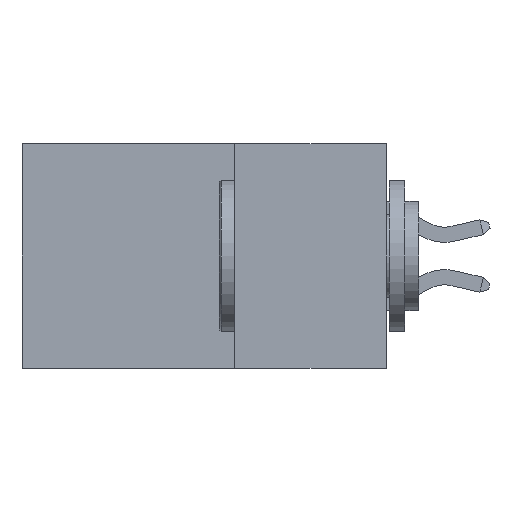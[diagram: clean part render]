
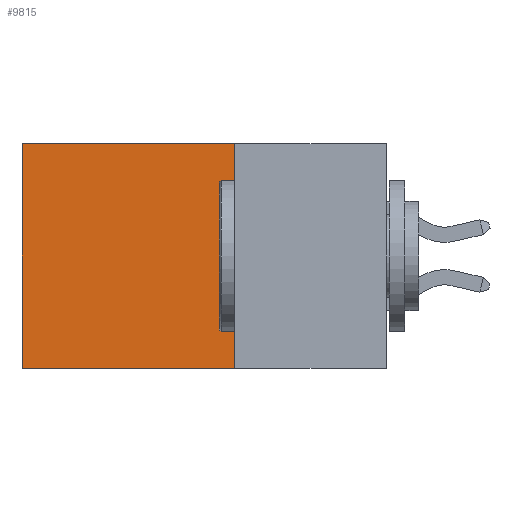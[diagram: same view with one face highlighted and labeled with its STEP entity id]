
A CAD part, left-side view. The second image highlights one B-rep face of the part: STEP entity #9815.
In plain terms, the highlighted planar face has unit normal (-1, 0, 0).
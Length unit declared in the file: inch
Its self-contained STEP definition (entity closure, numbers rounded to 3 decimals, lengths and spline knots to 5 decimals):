
#515 = EDGE_LOOP ( 'NONE', ( #5814, #2212, #3972, #2820 ) ) ;
#519 = DIRECTION ( 'NONE',  ( 0., 0., -1. ) ) ;
#528 = DIRECTION ( 'NONE',  ( 1., 0., 0. ) ) ;
#557 = CARTESIAN_POINT ( 'NONE',  ( 0.298, 0.25, 0. ) ) ;
#653 = PLANE ( 'NONE',  #1345 ) ;
#696 = LINE ( 'NONE', #3152, #5235 ) ;
#751 = LINE ( 'NONE', #9709, #7379 ) ;
#1121 = VERTEX_POINT ( 'NONE', #5261 ) ;
#1345 = AXIS2_PLACEMENT_3D ( 'NONE', #557, #528, #519 ) ;
#1665 = VERTEX_POINT ( 'NONE', #6172 ) ;
#1798 = DIRECTION ( 'NONE',  ( 0., 1., 0. ) ) ;
#1944 = CARTESIAN_POINT ( 'NONE',  ( 0.298, 0.25, 0. ) ) ;
#2212 = ORIENTED_EDGE ( 'NONE', *, *, #5221, .F. ) ;
#2407 = CARTESIAN_POINT ( 'NONE',  ( 0.298, 0.25, -0.37 ) ) ;
#2743 = VERTEX_POINT ( 'NONE', #1944 ) ;
#2820 = ORIENTED_EDGE ( 'NONE', *, *, #8321, .T. ) ;
#3152 = CARTESIAN_POINT ( 'NONE',  ( 0.298, 0.6, 0. ) ) ;
#3344 = FACE_OUTER_BOUND ( 'NONE', #515, .T. ) ;
#3363 = LINE ( 'NONE', #10147, #5412 ) ;
#3441 = CARTESIAN_POINT ( 'NONE',  ( 0.298, 0.6, 0. ) ) ;
#3619 = VECTOR ( 'NONE', #1798, 39.37008 ) ;
#3972 = ORIENTED_EDGE ( 'NONE', *, *, #4378, .F. ) ;
#4378 = EDGE_CURVE ( 'NONE', #2743, #1121, #3363, .T. ) ;
#5221 = EDGE_CURVE ( 'NONE', #1121, #1665, #5945, .T. ) ;
#5235 = VECTOR ( 'NONE', #9187, 39.37008 ) ;
#5261 = CARTESIAN_POINT ( 'NONE',  ( 0.298, 0.25, -0.37 ) ) ;
#5412 = VECTOR ( 'NONE', #9685, 39.37008 ) ;
#5814 = ORIENTED_EDGE ( 'NONE', *, *, #10454, .T. ) ;
#5945 = LINE ( 'NONE', #2407, #3619 ) ;
#6172 = CARTESIAN_POINT ( 'NONE',  ( 0.298, 0.6, -0.37 ) ) ;
#7379 = VECTOR ( 'NONE', #9727, 39.37008 ) ;
#8321 = EDGE_CURVE ( 'NONE', #2743, #9375, #751, .T. ) ;
#9187 = DIRECTION ( 'NONE',  ( 0., 0., -1. ) ) ;
#9375 = VERTEX_POINT ( 'NONE', #3441 ) ;
#9685 = DIRECTION ( 'NONE',  ( 0., 0., -1. ) ) ;
#9709 = CARTESIAN_POINT ( 'NONE',  ( 0.298, 0.25, 0. ) ) ;
#9727 = DIRECTION ( 'NONE',  ( 0., 1., 0. ) ) ;
#9815 = ADVANCED_FACE ( 'NONE', ( #3344 ), #653, .F. ) ;
#10147 = CARTESIAN_POINT ( 'NONE',  ( 0.298, 0.25, 0. ) ) ;
#10454 = EDGE_CURVE ( 'NONE', #9375, #1665, #696, .T. ) ;
